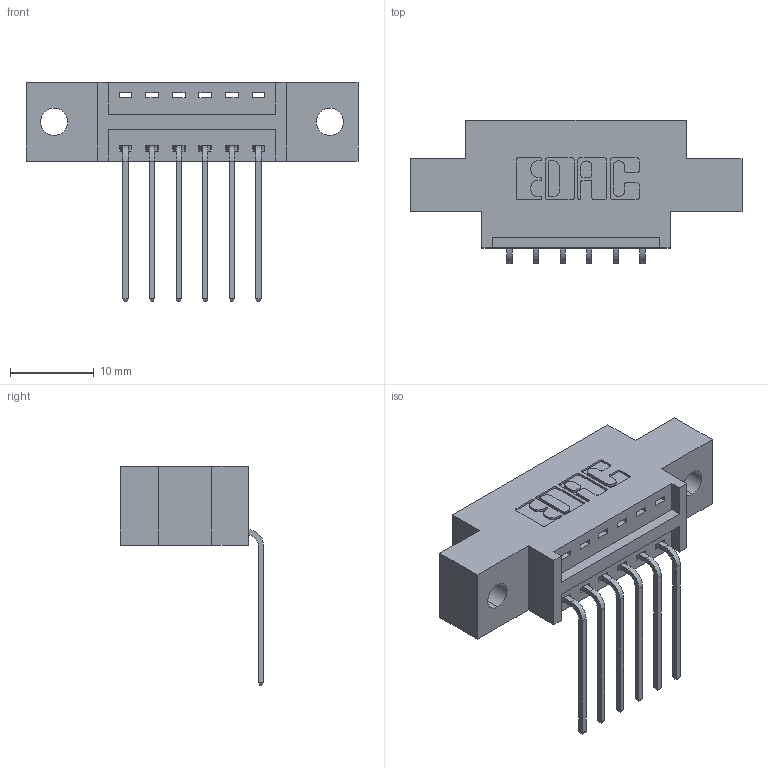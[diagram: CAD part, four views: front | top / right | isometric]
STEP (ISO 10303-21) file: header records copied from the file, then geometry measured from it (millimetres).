
FILE_DESCRIPTION (( 'STEP AP203' ), '1' );
FILE_NAME ('396-006-559-602.STEP', '2018-08-30T23:21:11', ( '' ), ( '' ), 'SwSTEP 2.0', 'SolidWorks 2016', '' );
FILE_SCHEMA (( 'CONFIG_CONTROL_DESIGN' ));
Length unit declared in the file: inch
Products named in the file (3): 346 Part_0.170 Offset - 0.128 Dia; 345-292-001_558 559 Tail - 1; 396-006-559-602
Assembly tree (7 placements, depth 2):
  396-006-559-602
    346 Part_0.170 Offset - 0.128 Dia
    345-292-001_558 559 Tail - 1  x6
Bounding box: 39.62 x 17.08 x 26.16 mm (x, y, z)
Volume: 3373.6 mm3; surface area: 3836.4 mm2
Topology: 7 solids, 7 shells, 486 faces, 1433 edges, 946 vertices
Faces by surface type: plane 332, cylinder 154
Entity records: 8789 total; most frequent: CARTESIAN_POINT 1526, ORIENTED_EDGE 1466, DIRECTION 1389, EDGE_CURVE 733, VECTOR 577, LINE 577, VERTEX_POINT 486, AXIS2_PLACEMENT_3D 406
